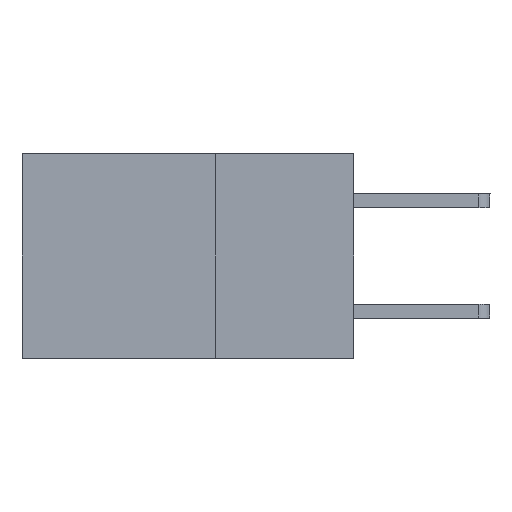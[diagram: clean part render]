
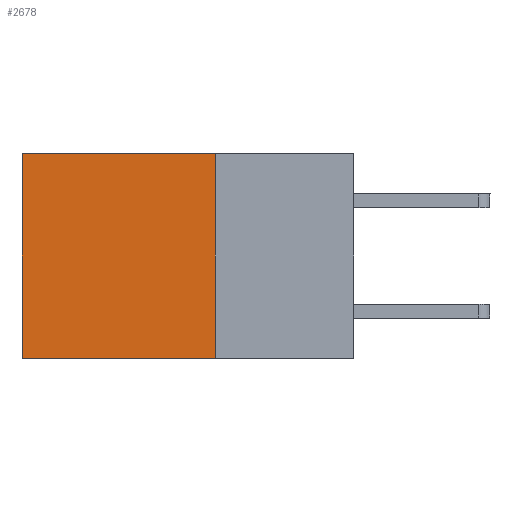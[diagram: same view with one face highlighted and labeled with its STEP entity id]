
A CAD part, left-side view. The second image highlights one B-rep face of the part: STEP entity #2678.
In plain terms, the highlighted planar face has unit normal (-1, 0, 0).
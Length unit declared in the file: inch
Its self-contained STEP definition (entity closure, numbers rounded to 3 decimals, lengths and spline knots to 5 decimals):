
#176 = VECTOR ( 'NONE', #11814, 39.37008 ) ;
#1015 = DIRECTION ( 'NONE',  ( 0., 1., 0. ) ) ;
#1090 = CARTESIAN_POINT ( 'NONE',  ( 0.2875, 0.6, -0.37 ) ) ;
#1124 = ORIENTED_EDGE ( 'NONE', *, *, #10921, .T. ) ;
#1188 = ORIENTED_EDGE ( 'NONE', *, *, #10643, .F. ) ;
#1239 = ORIENTED_EDGE ( 'NONE', *, *, #8775, .F. ) ;
#1350 = ORIENTED_EDGE ( 'NONE', *, *, #14197, .T. ) ;
#1903 = DIRECTION ( 'NONE',  ( 1., 0., 0. ) ) ;
#2139 = VECTOR ( 'NONE', #9892, 39.37008 ) ;
#2678 = ADVANCED_FACE ( 'NONE', ( #12461 ), #8721, .F. ) ;
#3081 = VECTOR ( 'NONE', #1015, 39.37008 ) ;
#3160 = CARTESIAN_POINT ( 'NONE',  ( 0.2875, 0.25, 0. ) ) ;
#5117 = VERTEX_POINT ( 'NONE', #1090 ) ;
#5468 = DIRECTION ( 'NONE',  ( 0., 1., 0. ) ) ;
#5601 = CARTESIAN_POINT ( 'NONE',  ( 0.2875, 0.6, 0. ) ) ;
#6324 = VERTEX_POINT ( 'NONE', #5601 ) ;
#6441 = EDGE_LOOP ( 'NONE', ( #1124, #1188, #1239, #1350 ) ) ;
#6720 = CARTESIAN_POINT ( 'NONE',  ( 0.2875, 0.25, 0. ) ) ;
#7036 = AXIS2_PLACEMENT_3D ( 'NONE', #11956, #1903, #9821 ) ;
#7244 = LINE ( 'NONE', #12165, #13114 ) ;
#8189 = LINE ( 'NONE', #3160, #2139 ) ;
#8721 = PLANE ( 'NONE',  #7036 ) ;
#8775 = EDGE_CURVE ( 'NONE', #13999, #13913, #8189, .T. ) ;
#9357 = LINE ( 'NONE', #13988, #176 ) ;
#9821 = DIRECTION ( 'NONE',  ( 0., 0., -1. ) ) ;
#9892 = DIRECTION ( 'NONE',  ( 0., 0., -1. ) ) ;
#10643 = EDGE_CURVE ( 'NONE', #13913, #5117, #7244, .T. ) ;
#10724 = CARTESIAN_POINT ( 'NONE',  ( 0.2875, 0.25, -0.37 ) ) ;
#10921 = EDGE_CURVE ( 'NONE', #6324, #5117, #9357, .T. ) ;
#11679 = LINE ( 'NONE', #6720, #3081 ) ;
#11814 = DIRECTION ( 'NONE',  ( 0., 0., -1. ) ) ;
#11956 = CARTESIAN_POINT ( 'NONE',  ( 0.2875, 0.25, 0. ) ) ;
#12165 = CARTESIAN_POINT ( 'NONE',  ( 0.2875, 0.25, -0.37 ) ) ;
#12461 = FACE_OUTER_BOUND ( 'NONE', #6441, .T. ) ;
#13114 = VECTOR ( 'NONE', #5468, 39.37008 ) ;
#13913 = VERTEX_POINT ( 'NONE', #10724 ) ;
#13988 = CARTESIAN_POINT ( 'NONE',  ( 0.2875, 0.6, 0. ) ) ;
#13999 = VERTEX_POINT ( 'NONE', #14107 ) ;
#14107 = CARTESIAN_POINT ( 'NONE',  ( 0.2875, 0.25, 0. ) ) ;
#14197 = EDGE_CURVE ( 'NONE', #13999, #6324, #11679, .T. ) ;
